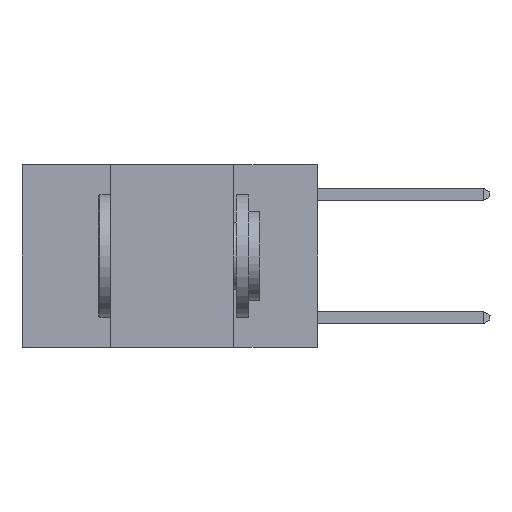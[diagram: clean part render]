
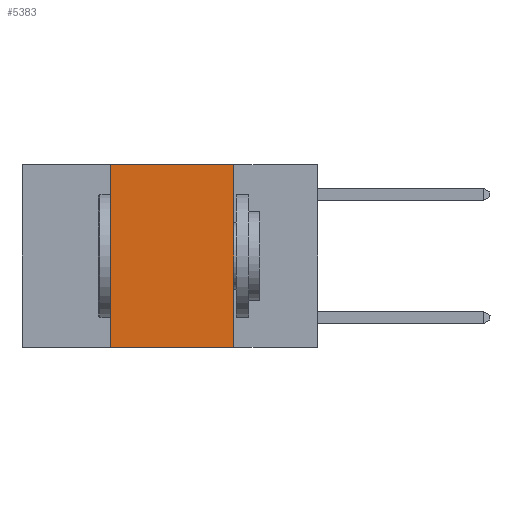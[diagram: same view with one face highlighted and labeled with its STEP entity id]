
A CAD part, left-side view. The second image highlights one B-rep face of the part: STEP entity #5383.
In plain terms, the highlighted planar face has unit normal (-1, 0, 0).
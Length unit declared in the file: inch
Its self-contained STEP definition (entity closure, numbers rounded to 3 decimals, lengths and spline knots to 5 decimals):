
#1 = ORIENTED_EDGE ( 'NONE', *, *, #21133, .F. ) ;
#895 = VERTEX_POINT ( 'NONE', #7303 ) ;
#1288 = LINE ( 'NONE', #15610, #20467 ) ;
#2892 = DIRECTION ( 'NONE',  ( 0., 0., -1. ) ) ;
#3769 = VERTEX_POINT ( 'NONE', #24703 ) ;
#4180 = LINE ( 'NONE', #12034, #22340 ) ;
#4406 = DIRECTION ( 'NONE',  ( 0., 0., 1. ) ) ;
#4814 = CARTESIAN_POINT ( 'NONE',  ( 0., 0.6, 0. ) ) ;
#5191 = EDGE_CURVE ( 'NONE', #3769, #11579, #25398, .T. ) ;
#5383 = ADVANCED_FACE ( 'NONE', ( #19942 ), #19538, .F. ) ;
#5438 = AXIS2_PLACEMENT_3D ( 'NONE', #4814, #15416, #2892 ) ;
#5698 = CARTESIAN_POINT ( 'NONE',  ( 0., 0.42, 0. ) ) ;
#5910 = EDGE_CURVE ( 'NONE', #11579, #7707, #16614, .T. ) ;
#6094 = ORIENTED_EDGE ( 'NONE', *, *, #5191, .F. ) ;
#7303 = CARTESIAN_POINT ( 'NONE',  ( 0., 0.17, -0.37 ) ) ;
#7707 = VERTEX_POINT ( 'NONE', #15643 ) ;
#9832 = VECTOR ( 'NONE', #4406, 39.37008 ) ;
#10158 = DIRECTION ( 'NONE',  ( 0., -1., 0. ) ) ;
#11579 = VERTEX_POINT ( 'NONE', #5698 ) ;
#12034 = CARTESIAN_POINT ( 'NONE',  ( 0., 0.17, 0. ) ) ;
#12490 = CARTESIAN_POINT ( 'NONE',  ( 0., 0.6, 0. ) ) ;
#14473 = ORIENTED_EDGE ( 'NONE', *, *, #17217, .T. ) ;
#15416 = DIRECTION ( 'NONE',  ( 1., 0., 0. ) ) ;
#15610 = CARTESIAN_POINT ( 'NONE',  ( 0., 0.6, -0.37 ) ) ;
#15643 = CARTESIAN_POINT ( 'NONE',  ( 0., 0.17, 0. ) ) ;
#16172 = DIRECTION ( 'NONE',  ( 0., 0., -1. ) ) ;
#16614 = LINE ( 'NONE', #12490, #17314 ) ;
#17217 = EDGE_CURVE ( 'NONE', #3769, #895, #1288, .T. ) ;
#17314 = VECTOR ( 'NONE', #10158, 39.37008 ) ;
#17665 = DIRECTION ( 'NONE',  ( 0., -1., 0. ) ) ;
#18862 = CARTESIAN_POINT ( 'NONE',  ( 0., 0.42, 0. ) ) ;
#19538 = PLANE ( 'NONE',  #5438 ) ;
#19942 = FACE_OUTER_BOUND ( 'NONE', #20984, .T. ) ;
#20467 = VECTOR ( 'NONE', #17665, 39.37008 ) ;
#20984 = EDGE_LOOP ( 'NONE', ( #1, #23569, #6094, #14473 ) ) ;
#21133 = EDGE_CURVE ( 'NONE', #7707, #895, #4180, .T. ) ;
#22340 = VECTOR ( 'NONE', #16172, 39.37008 ) ;
#23569 = ORIENTED_EDGE ( 'NONE', *, *, #5910, .F. ) ;
#24703 = CARTESIAN_POINT ( 'NONE',  ( 0., 0.42, -0.37 ) ) ;
#25398 = LINE ( 'NONE', #18862, #9832 ) ;
